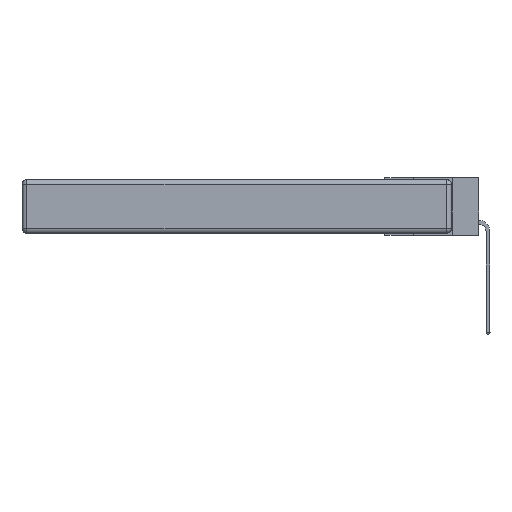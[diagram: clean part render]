
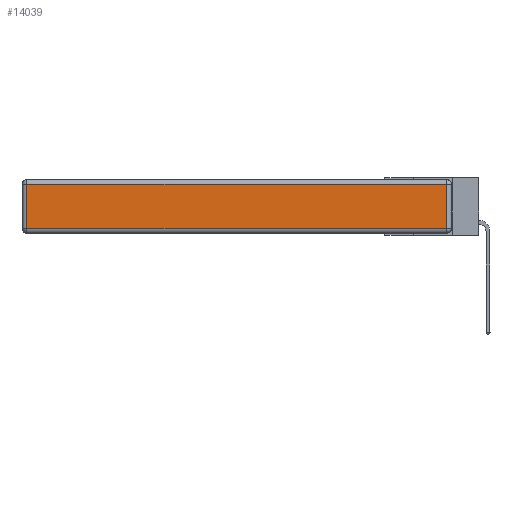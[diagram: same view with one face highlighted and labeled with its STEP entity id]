
A CAD part, left-side view. The second image highlights one B-rep face of the part: STEP entity #14039.
In plain terms, the highlighted planar face has unit normal (-1, 0, 0).
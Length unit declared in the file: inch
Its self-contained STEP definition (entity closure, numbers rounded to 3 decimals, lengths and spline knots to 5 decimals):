
#805 = CARTESIAN_POINT ( 'NONE',  ( 0., 2.72, -0.343 ) ) ;
#862 = CARTESIAN_POINT ( 'NONE',  ( 0., 0.03, -0.03 ) ) ;
#1036 = VECTOR ( 'NONE', #2706, 39.37008 ) ;
#2706 = DIRECTION ( 'NONE',  ( 0., 1., 0. ) ) ;
#4645 = EDGE_CURVE ( 'NONE', #14326, #7764, #15036, .T. ) ;
#4662 = ORIENTED_EDGE ( 'NONE', *, *, #25553, .T. ) ;
#4709 = VECTOR ( 'NONE', #25211, 39.37008 ) ;
#7427 = DIRECTION ( 'NONE',  ( 0., 0., 1. ) ) ;
#7764 = VERTEX_POINT ( 'NONE', #28594 ) ;
#8730 = DIRECTION ( 'NONE',  ( 0., 0., 1. ) ) ;
#9328 = FACE_OUTER_BOUND ( 'NONE', #22878, .T. ) ;
#9361 = VERTEX_POINT ( 'NONE', #862 ) ;
#9583 = CARTESIAN_POINT ( 'NONE',  ( 0., 2.75, -0.03 ) ) ;
#9663 = CARTESIAN_POINT ( 'NONE',  ( 0., 0.03, -0.313 ) ) ;
#10311 = VERTEX_POINT ( 'NONE', #9663 ) ;
#10592 = CARTESIAN_POINT ( 'NONE',  ( 0., 0.03, -0.343 ) ) ;
#10756 = ORIENTED_EDGE ( 'NONE', *, *, #18757, .T. ) ;
#11570 = LINE ( 'NONE', #26056, #27283 ) ;
#14039 = ADVANCED_FACE ( 'NONE', ( #9328 ), #22106, .T. ) ;
#14130 = CARTESIAN_POINT ( 'NONE',  ( 0., 2.72, -0.03 ) ) ;
#14326 = VERTEX_POINT ( 'NONE', #14130 ) ;
#14706 = DIRECTION ( 'NONE',  ( -1., 0., 0. ) ) ;
#15017 = CARTESIAN_POINT ( 'NONE',  ( 0., 0., -0.343 ) ) ;
#15036 = LINE ( 'NONE', #805, #4709 ) ;
#16337 = LINE ( 'NONE', #9583, #1036 ) ;
#17387 = ORIENTED_EDGE ( 'NONE', *, *, #4645, .T. ) ;
#18168 = AXIS2_PLACEMENT_3D ( 'NONE', #15017, #14706, #7427 ) ;
#18757 = EDGE_CURVE ( 'NONE', #10311, #9361, #23818, .T. ) ;
#20564 = ORIENTED_EDGE ( 'NONE', *, *, #22376, .T. ) ;
#20985 = DIRECTION ( 'NONE',  ( 0., -1., 0. ) ) ;
#22106 = PLANE ( 'NONE',  #18168 ) ;
#22376 = EDGE_CURVE ( 'NONE', #7764, #10311, #11570, .T. ) ;
#22878 = EDGE_LOOP ( 'NONE', ( #20564, #10756, #4662, #17387 ) ) ;
#23818 = LINE ( 'NONE', #10592, #27655 ) ;
#25211 = DIRECTION ( 'NONE',  ( 0., 0., -1. ) ) ;
#25553 = EDGE_CURVE ( 'NONE', #9361, #14326, #16337, .T. ) ;
#26056 = CARTESIAN_POINT ( 'NONE',  ( 0., 0., -0.313 ) ) ;
#27283 = VECTOR ( 'NONE', #20985, 39.37008 ) ;
#27655 = VECTOR ( 'NONE', #8730, 39.37008 ) ;
#28594 = CARTESIAN_POINT ( 'NONE',  ( 0., 2.72, -0.313 ) ) ;
